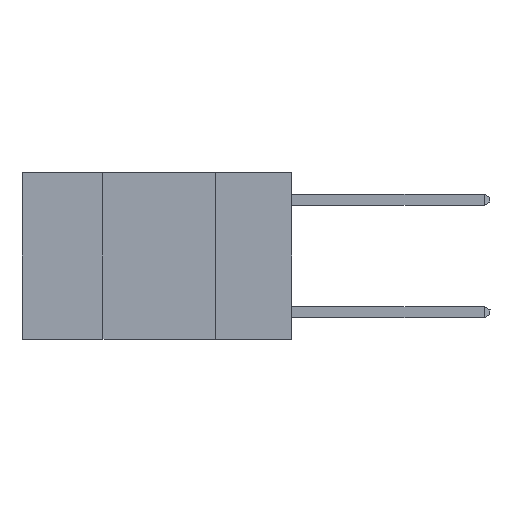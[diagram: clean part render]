
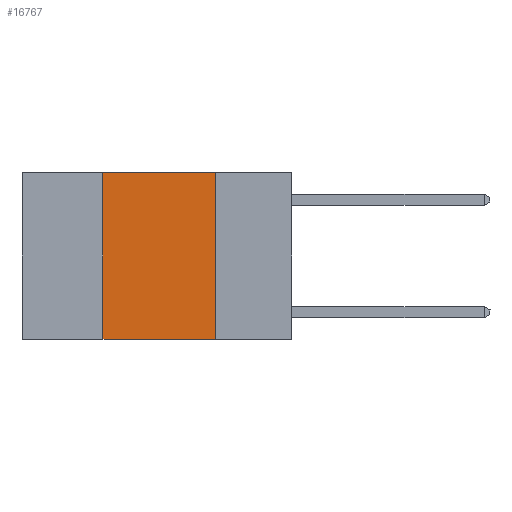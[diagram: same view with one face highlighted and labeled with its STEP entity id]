
A CAD part, left-side view. The second image highlights one B-rep face of the part: STEP entity #16767.
In plain terms, the highlighted planar face has unit normal (-1, 0, 0).
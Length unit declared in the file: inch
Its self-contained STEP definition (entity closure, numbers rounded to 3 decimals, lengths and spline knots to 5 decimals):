
#1196 = DIRECTION ( 'NONE',  ( 1., 0., 0. ) ) ;
#1565 = VERTEX_POINT ( 'NONE', #31485 ) ;
#2196 = VECTOR ( 'NONE', #26163, 39.37008 ) ;
#2495 = LINE ( 'NONE', #10125, #7089 ) ;
#2947 = DIRECTION ( 'NONE',  ( 0., 0., 1. ) ) ;
#3782 = VERTEX_POINT ( 'NONE', #24722 ) ;
#4027 = DIRECTION ( 'NONE',  ( 0., 0., -1. ) ) ;
#6622 = LINE ( 'NONE', #16134, #20914 ) ;
#7089 = VECTOR ( 'NONE', #24956, 39.37008 ) ;
#8248 = CARTESIAN_POINT ( 'NONE',  ( 0., 0.42, 0. ) ) ;
#8898 = CARTESIAN_POINT ( 'NONE',  ( 0., 0.17, -0.37 ) ) ;
#9110 = VERTEX_POINT ( 'NONE', #13791 ) ;
#9655 = EDGE_CURVE ( 'NONE', #9110, #3782, #18910, .T. ) ;
#9938 = VECTOR ( 'NONE', #2947, 39.37008 ) ;
#10125 = CARTESIAN_POINT ( 'NONE',  ( 0., 0.6, 0. ) ) ;
#11818 = CARTESIAN_POINT ( 'NONE',  ( 0., 0.6, 0. ) ) ;
#12595 = ORIENTED_EDGE ( 'NONE', *, *, #28890, .F. ) ;
#13791 = CARTESIAN_POINT ( 'NONE',  ( 0., 0.42, -0.37 ) ) ;
#13989 = EDGE_CURVE ( 'NONE', #9110, #14518, #6622, .T. ) ;
#14518 = VERTEX_POINT ( 'NONE', #8898 ) ;
#15836 = CARTESIAN_POINT ( 'NONE',  ( 0., 0.17, 0. ) ) ;
#15992 = LINE ( 'NONE', #15836, #2196 ) ;
#16134 = CARTESIAN_POINT ( 'NONE',  ( 0., 0.6, -0.37 ) ) ;
#16767 = ADVANCED_FACE ( 'NONE', ( #21347 ), #31881, .F. ) ;
#18910 = LINE ( 'NONE', #8248, #9938 ) ;
#19338 = AXIS2_PLACEMENT_3D ( 'NONE', #11818, #1196, #4027 ) ;
#20914 = VECTOR ( 'NONE', #26324, 39.37008 ) ;
#21347 = FACE_OUTER_BOUND ( 'NONE', #31560, .T. ) ;
#21958 = ORIENTED_EDGE ( 'NONE', *, *, #13989, .T. ) ;
#24302 = ORIENTED_EDGE ( 'NONE', *, *, #24778, .F. ) ;
#24722 = CARTESIAN_POINT ( 'NONE',  ( 0., 0.42, 0. ) ) ;
#24778 = EDGE_CURVE ( 'NONE', #3782, #1565, #2495, .T. ) ;
#24956 = DIRECTION ( 'NONE',  ( 0., -1., 0. ) ) ;
#26163 = DIRECTION ( 'NONE',  ( 0., 0., -1. ) ) ;
#26324 = DIRECTION ( 'NONE',  ( 0., -1., 0. ) ) ;
#28890 = EDGE_CURVE ( 'NONE', #1565, #14518, #15992, .T. ) ;
#29918 = ORIENTED_EDGE ( 'NONE', *, *, #9655, .F. ) ;
#31485 = CARTESIAN_POINT ( 'NONE',  ( 0., 0.17, 0. ) ) ;
#31560 = EDGE_LOOP ( 'NONE', ( #12595, #24302, #29918, #21958 ) ) ;
#31881 = PLANE ( 'NONE',  #19338 ) ;
